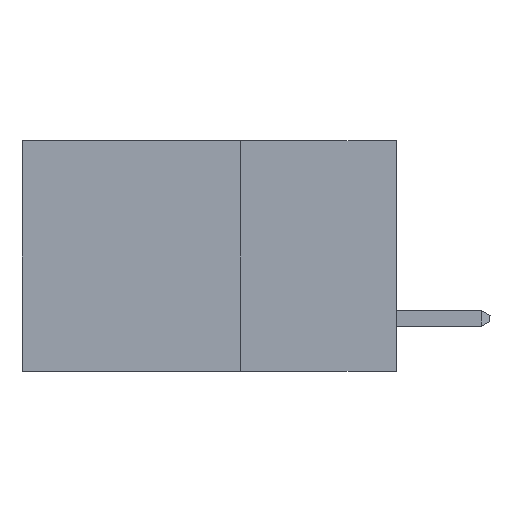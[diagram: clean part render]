
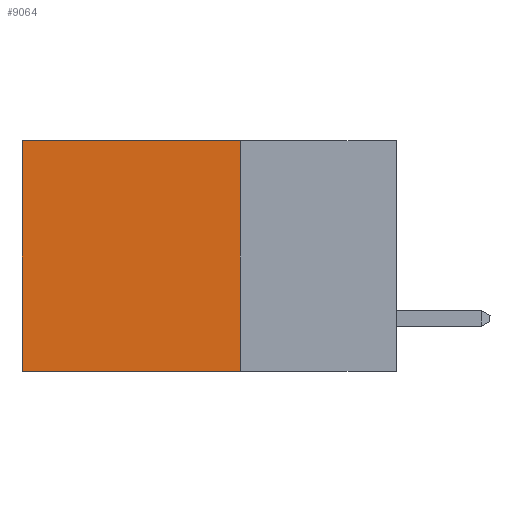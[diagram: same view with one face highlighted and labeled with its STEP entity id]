
A CAD part, left-side view. The second image highlights one B-rep face of the part: STEP entity #9064.
In plain terms, the highlighted planar face has unit normal (-1, 0, 0).
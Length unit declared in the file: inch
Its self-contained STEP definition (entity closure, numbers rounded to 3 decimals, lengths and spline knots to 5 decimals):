
#669 = ORIENTED_EDGE ( 'NONE', *, *, #10632, .T. ) ;
#892 = VECTOR ( 'NONE', #9175, 39.37008 ) ;
#918 = CARTESIAN_POINT ( 'NONE',  ( 0.2615, 0.6, -0.37 ) ) ;
#976 = PLANE ( 'NONE',  #11819 ) ;
#995 = CARTESIAN_POINT ( 'NONE',  ( 0.2615, 0.25, -0.37 ) ) ;
#998 = LINE ( 'NONE', #10146, #892 ) ;
#1208 = ORIENTED_EDGE ( 'NONE', *, *, #11906, .F. ) ;
#2658 = EDGE_CURVE ( 'NONE', #6979, #9840, #5186, .T. ) ;
#2817 = DIRECTION ( 'NONE',  ( 0., 1., 0. ) ) ;
#3217 = CARTESIAN_POINT ( 'NONE',  ( 0.2615, 0.25, 0. ) ) ;
#3507 = VECTOR ( 'NONE', #2817, 39.37008 ) ;
#3565 = VECTOR ( 'NONE', #4992, 39.37008 ) ;
#3911 = CARTESIAN_POINT ( 'NONE',  ( 0.2615, 0.6, 0. ) ) ;
#4024 = EDGE_CURVE ( 'NONE', #6979, #11166, #998, .T. ) ;
#4728 = LINE ( 'NONE', #918, #5804 ) ;
#4992 = DIRECTION ( 'NONE',  ( 0., 0., -1. ) ) ;
#5141 = CARTESIAN_POINT ( 'NONE',  ( 0.2615, 0.25, -0.37 ) ) ;
#5186 = LINE ( 'NONE', #995, #3565 ) ;
#5516 = ORIENTED_EDGE ( 'NONE', *, *, #4024, .T. ) ;
#5804 = VECTOR ( 'NONE', #10725, 39.37008 ) ;
#5893 = FACE_OUTER_BOUND ( 'NONE', #12575, .T. ) ;
#6730 = CARTESIAN_POINT ( 'NONE',  ( 0.2615, 0.6, -0.37 ) ) ;
#6979 = VERTEX_POINT ( 'NONE', #3217 ) ;
#8962 = DIRECTION ( 'NONE',  ( 0., 0., -1. ) ) ;
#9064 = ADVANCED_FACE ( 'NONE', ( #5893 ), #976, .F. ) ;
#9175 = DIRECTION ( 'NONE',  ( 0., 1., 0. ) ) ;
#9743 = DIRECTION ( 'NONE',  ( 1., 0., 0. ) ) ;
#9755 = CARTESIAN_POINT ( 'NONE',  ( 0.2615, 0.25, -0.37 ) ) ;
#9840 = VERTEX_POINT ( 'NONE', #5141 ) ;
#10146 = CARTESIAN_POINT ( 'NONE',  ( 0.2615, 0.25, 0. ) ) ;
#10632 = EDGE_CURVE ( 'NONE', #11166, #12421, #4728, .T. ) ;
#10725 = DIRECTION ( 'NONE',  ( 0., 0., -1. ) ) ;
#11166 = VERTEX_POINT ( 'NONE', #3911 ) ;
#11607 = ORIENTED_EDGE ( 'NONE', *, *, #2658, .F. ) ;
#11819 = AXIS2_PLACEMENT_3D ( 'NONE', #12874, #9743, #8962 ) ;
#11906 = EDGE_CURVE ( 'NONE', #9840, #12421, #12693, .T. ) ;
#12421 = VERTEX_POINT ( 'NONE', #6730 ) ;
#12575 = EDGE_LOOP ( 'NONE', ( #669, #1208, #11607, #5516 ) ) ;
#12693 = LINE ( 'NONE', #9755, #3507 ) ;
#12874 = CARTESIAN_POINT ( 'NONE',  ( 0.2615, 0.25, -0.37 ) ) ;
